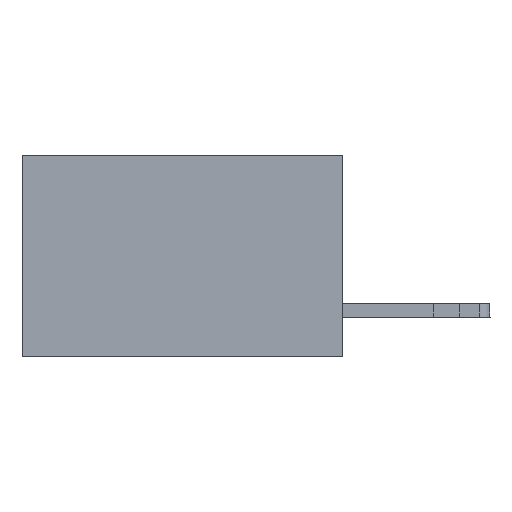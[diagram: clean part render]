
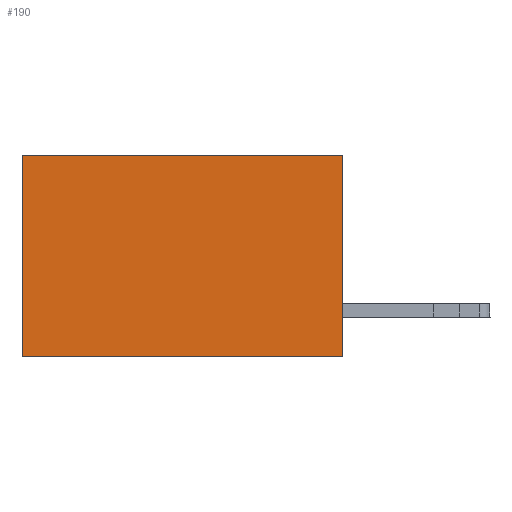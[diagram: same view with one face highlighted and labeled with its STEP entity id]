
A CAD part, left-side view. The second image highlights one B-rep face of the part: STEP entity #190.
In plain terms, the highlighted planar face has unit normal (-1, 0, 0).
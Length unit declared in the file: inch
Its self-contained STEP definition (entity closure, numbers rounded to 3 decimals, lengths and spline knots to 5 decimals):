
#190 = ADVANCED_FACE ( 'NONE', ( #6145 ), #14360, .F. ) ;
#213 = DIRECTION ( 'NONE',  ( 1., 0., 0. ) ) ;
#274 = CARTESIAN_POINT ( 'NONE',  ( 0.277, 0., 0. ) ) ;
#1019 = EDGE_CURVE ( 'NONE', #24009, #18036, #10489, .T. ) ;
#1446 = ORIENTED_EDGE ( 'NONE', *, *, #1019, .F. ) ;
#3248 = VECTOR ( 'NONE', #10222, 39.37008 ) ;
#3615 = VERTEX_POINT ( 'NONE', #6557 ) ;
#3738 = CARTESIAN_POINT ( 'NONE',  ( 0.277, 0.59, -0.37 ) ) ;
#3783 = EDGE_CURVE ( 'NONE', #3615, #18036, #15573, .T. ) ;
#5347 = VECTOR ( 'NONE', #22026, 39.37008 ) ;
#5841 = CARTESIAN_POINT ( 'NONE',  ( 0.277, 0., -0.37 ) ) ;
#5920 = CARTESIAN_POINT ( 'NONE',  ( 0.277, 0.59, -0.37 ) ) ;
#6145 = FACE_OUTER_BOUND ( 'NONE', #9721, .T. ) ;
#6557 = CARTESIAN_POINT ( 'NONE',  ( 0.277, 0.59, 0. ) ) ;
#9620 = EDGE_CURVE ( 'NONE', #13555, #3615, #15678, .T. ) ;
#9721 = EDGE_LOOP ( 'NONE', ( #11472, #1446, #12885, #13994 ) ) ;
#10222 = DIRECTION ( 'NONE',  ( 0., 1., 0. ) ) ;
#10489 = LINE ( 'NONE', #20889, #3248 ) ;
#11472 = ORIENTED_EDGE ( 'NONE', *, *, #3783, .T. ) ;
#12885 = ORIENTED_EDGE ( 'NONE', *, *, #15561, .F. ) ;
#13507 = LINE ( 'NONE', #5841, #5347 ) ;
#13555 = VERTEX_POINT ( 'NONE', #274 ) ;
#13810 = DIRECTION ( 'NONE',  ( 0., 0., -1. ) ) ;
#13994 = ORIENTED_EDGE ( 'NONE', *, *, #9620, .T. ) ;
#14360 = PLANE ( 'NONE',  #16152 ) ;
#15561 = EDGE_CURVE ( 'NONE', #13555, #24009, #13507, .T. ) ;
#15573 = LINE ( 'NONE', #3738, #17329 ) ;
#15678 = LINE ( 'NONE', #26335, #19398 ) ;
#16152 = AXIS2_PLACEMENT_3D ( 'NONE', #24368, #213, #22608 ) ;
#17329 = VECTOR ( 'NONE', #13810, 39.37008 ) ;
#18036 = VERTEX_POINT ( 'NONE', #5920 ) ;
#19398 = VECTOR ( 'NONE', #19865, 39.37008 ) ;
#19708 = CARTESIAN_POINT ( 'NONE',  ( 0.277, 0., -0.37 ) ) ;
#19865 = DIRECTION ( 'NONE',  ( 0., 1., 0. ) ) ;
#20889 = CARTESIAN_POINT ( 'NONE',  ( 0.277, 0., -0.37 ) ) ;
#22026 = DIRECTION ( 'NONE',  ( 0., 0., -1. ) ) ;
#22608 = DIRECTION ( 'NONE',  ( 0., 0., -1. ) ) ;
#24009 = VERTEX_POINT ( 'NONE', #19708 ) ;
#24368 = CARTESIAN_POINT ( 'NONE',  ( 0.277, 0., -0.37 ) ) ;
#26335 = CARTESIAN_POINT ( 'NONE',  ( 0.277, 0., 0. ) ) ;
